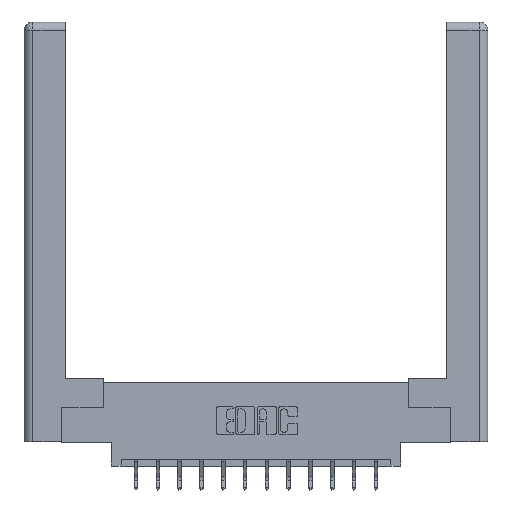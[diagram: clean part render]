
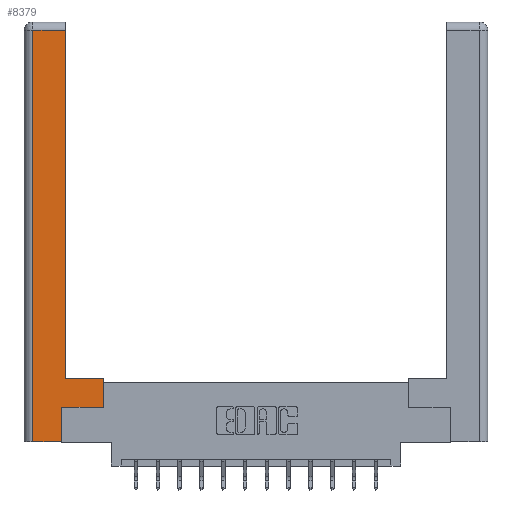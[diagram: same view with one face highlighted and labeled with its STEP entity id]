
A CAD part, top view. The second image highlights one B-rep face of the part: STEP entity #8379.
In plain terms, the highlighted planar face has unit normal (0, 0, 1).
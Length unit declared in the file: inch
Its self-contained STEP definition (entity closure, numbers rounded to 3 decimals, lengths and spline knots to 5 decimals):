
#269 = VECTOR ( 'NONE', #791, 39.37008 ) ;
#431 = CARTESIAN_POINT ( 'NONE',  ( 0.295, 3., 0. ) ) ;
#578 = VERTEX_POINT ( 'NONE', #9939 ) ;
#791 = DIRECTION ( 'NONE',  ( 0., 1., 0. ) ) ;
#994 = CARTESIAN_POINT ( 'NONE',  ( 0.0615, 2.94, 0. ) ) ;
#1022 = LINE ( 'NONE', #2705, #1433 ) ;
#1036 = CARTESIAN_POINT ( 'NONE',  ( 0.565, 0.245, 0. ) ) ;
#1355 = CARTESIAN_POINT ( 'NONE',  ( 0.265, 0.245, 0. ) ) ;
#1433 = VECTOR ( 'NONE', #11410, 39.37008 ) ;
#1435 = EDGE_CURVE ( 'NONE', #13923, #8370, #10963, .T. ) ;
#1588 = VECTOR ( 'NONE', #15727, 39.37008 ) ;
#1869 = LINE ( 'NONE', #3971, #9689 ) ;
#2641 = VERTEX_POINT ( 'NONE', #11047 ) ;
#2705 = CARTESIAN_POINT ( 'NONE',  ( 0.565, 0.245, 0. ) ) ;
#3000 = ORIENTED_EDGE ( 'NONE', *, *, #5947, .T. ) ;
#3274 = ORIENTED_EDGE ( 'NONE', *, *, #7190, .T. ) ;
#3716 = ORIENTED_EDGE ( 'NONE', *, *, #10150, .T. ) ;
#3964 = DIRECTION ( 'NONE',  ( 0., -1., 0. ) ) ;
#3971 = CARTESIAN_POINT ( 'NONE',  ( 0.295, 0.45, 0. ) ) ;
#4176 = CARTESIAN_POINT ( 'NONE',  ( 0.0615, 0., 0. ) ) ;
#4179 = ORIENTED_EDGE ( 'NONE', *, *, #8517, .T. ) ;
#5494 = CARTESIAN_POINT ( 'NONE',  ( 0.265, 0., 0. ) ) ;
#5947 = EDGE_CURVE ( 'NONE', #8653, #11228, #9633, .T. ) ;
#6515 = CARTESIAN_POINT ( 'NONE',  ( 0.0615, 0., 0. ) ) ;
#6878 = LINE ( 'NONE', #431, #1588 ) ;
#7190 = EDGE_CURVE ( 'NONE', #578, #13923, #6878, .T. ) ;
#7361 = DIRECTION ( 'NONE',  ( -1., 0., 0. ) ) ;
#7362 = CARTESIAN_POINT ( 'NONE',  ( 0.265, 0.245, 0. ) ) ;
#7523 = ORIENTED_EDGE ( 'NONE', *, *, #1435, .T. ) ;
#8370 = VERTEX_POINT ( 'NONE', #11870 ) ;
#8379 = ADVANCED_FACE ( 'NONE', ( #10278 ), #12039, .F. ) ;
#8474 = VERTEX_POINT ( 'NONE', #7362 ) ;
#8517 = EDGE_CURVE ( 'NONE', #11228, #578, #1869, .T. ) ;
#8653 = VERTEX_POINT ( 'NONE', #1036 ) ;
#9483 = CARTESIAN_POINT ( 'NONE',  ( 0.295, 2.94, 0. ) ) ;
#9580 = DIRECTION ( 'NONE',  ( 0., 0., -1. ) ) ;
#9633 = LINE ( 'NONE', #14509, #269 ) ;
#9689 = VECTOR ( 'NONE', #12878, 39.37008 ) ;
#9939 = CARTESIAN_POINT ( 'NONE',  ( 0.295, 0.45, 0. ) ) ;
#10116 = LINE ( 'NONE', #4176, #15589 ) ;
#10150 = EDGE_CURVE ( 'NONE', #2641, #8474, #10392, .T. ) ;
#10278 = FACE_OUTER_BOUND ( 'NONE', #14118, .T. ) ;
#10392 = LINE ( 'NONE', #1355, #11746 ) ;
#10486 = EDGE_CURVE ( 'NONE', #8474, #8653, #1022, .T. ) ;
#10963 = LINE ( 'NONE', #994, #11551 ) ;
#11047 = CARTESIAN_POINT ( 'NONE',  ( 0.265, 0., 0. ) ) ;
#11110 = AXIS2_PLACEMENT_3D ( 'NONE', #15824, #9580, #14398 ) ;
#11228 = VERTEX_POINT ( 'NONE', #12274 ) ;
#11410 = DIRECTION ( 'NONE',  ( 1., 0., 0. ) ) ;
#11551 = VECTOR ( 'NONE', #7361, 39.37008 ) ;
#11625 = VECTOR ( 'NONE', #13546, 39.37008 ) ;
#11746 = VECTOR ( 'NONE', #12361, 39.37008 ) ;
#11824 = ORIENTED_EDGE ( 'NONE', *, *, #12193, .T. ) ;
#11870 = CARTESIAN_POINT ( 'NONE',  ( 0.0615, 2.94, 0. ) ) ;
#12039 = PLANE ( 'NONE',  #11110 ) ;
#12193 = EDGE_CURVE ( 'NONE', #13603, #2641, #14992, .T. ) ;
#12274 = CARTESIAN_POINT ( 'NONE',  ( 0.565, 0.45, 0. ) ) ;
#12361 = DIRECTION ( 'NONE',  ( 0., 1., 0. ) ) ;
#12878 = DIRECTION ( 'NONE',  ( -1., 0., 0. ) ) ;
#13546 = DIRECTION ( 'NONE',  ( 1., 0., 0. ) ) ;
#13603 = VERTEX_POINT ( 'NONE', #6515 ) ;
#13674 = EDGE_CURVE ( 'NONE', #8370, #13603, #10116, .T. ) ;
#13923 = VERTEX_POINT ( 'NONE', #9483 ) ;
#14118 = EDGE_LOOP ( 'NONE', ( #3274, #7523, #14623, #11824, #3716, #16174, #3000, #4179 ) ) ;
#14398 = DIRECTION ( 'NONE',  ( -1., 0., 0. ) ) ;
#14509 = CARTESIAN_POINT ( 'NONE',  ( 0.565, 0.45, 0. ) ) ;
#14623 = ORIENTED_EDGE ( 'NONE', *, *, #13674, .T. ) ;
#14992 = LINE ( 'NONE', #5494, #11625 ) ;
#15589 = VECTOR ( 'NONE', #3964, 39.37008 ) ;
#15727 = DIRECTION ( 'NONE',  ( 0., 1., 0. ) ) ;
#15824 = CARTESIAN_POINT ( 'NONE',  ( 0., 0., 0. ) ) ;
#16174 = ORIENTED_EDGE ( 'NONE', *, *, #10486, .T. ) ;
